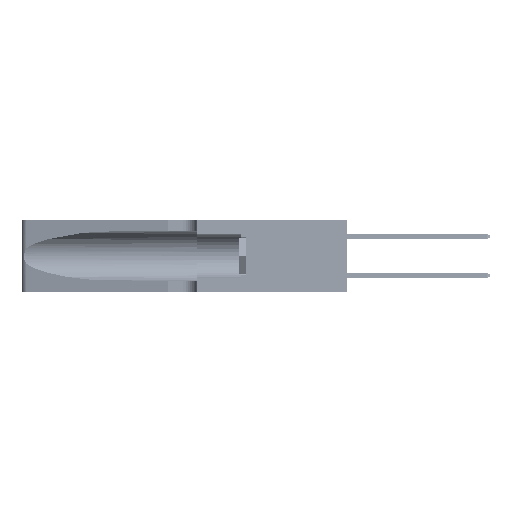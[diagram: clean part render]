
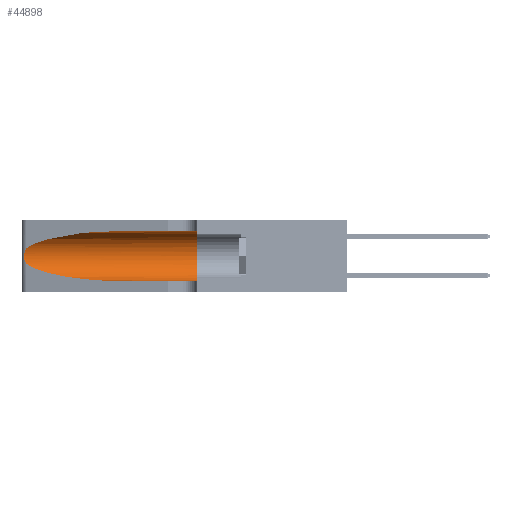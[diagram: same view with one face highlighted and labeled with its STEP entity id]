
A CAD part, left-side view. The second image highlights one B-rep face of the part: STEP entity #44898.
In plain terms, the highlighted cylindrical face has radius 3.308 mm (diameter 6.617 mm), a partial arc.
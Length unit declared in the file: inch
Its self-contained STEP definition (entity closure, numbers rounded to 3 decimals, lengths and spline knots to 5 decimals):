
#579 = CARTESIAN_POINT ( 'NONE',  ( 0.25487, 1.22718, 0.14631 ) ) ;
#1348 = CARTESIAN_POINT ( 'NONE',  ( 0.25487, 1.22718, 0.14631 ) ) ;
#1531 = CARTESIAN_POINT ( 'NONE',  ( 0.25639, 1.23184, 0.21858 ) ) ;
#1665 = EDGE_CURVE ( 'NONE', #18234, #7798, #29193, .T. ) ;
#2332 = ORIENTED_EDGE ( 'NONE', *, *, #12130, .F. ) ;
#2845 = CYLINDRICAL_SURFACE ( 'NONE', #19624, 0.13025 ) ;
#4830 = DIRECTION ( 'NONE',  ( 0., 1., 0. ) ) ;
#4990 = EDGE_CURVE ( 'NONE', #44279, #20820, #53232, .T. ) ;
#7434 = CARTESIAN_POINT ( 'NONE',  ( 0.1305, 1.61858, 0.185 ) ) ;
#7798 = VERTEX_POINT ( 'NONE', #15368 ) ;
#9820 = CARTESIAN_POINT ( 'NONE',  ( 0.26018, 1.23835, 0.19895 ) ) ;
#10367 = CARTESIAN_POINT ( 'NONE',  ( 0.1305, 0.35, 0.31525 ) ) ;
#10789 = CARTESIAN_POINT ( 'NONE',  ( 0.1305, 1.61858, 0.05475 ) ) ;
#12130 = EDGE_CURVE ( 'NONE', #43052, #50158, #14199, .T. ) ;
#13194 = CARTESIAN_POINT ( 'NONE',  ( 0.2373, 1.15595, 0.08982 ) ) ;
#13566 = CARTESIAN_POINT ( 'NONE',  ( 0.1305, 0.72297, 0.31525 ) ) ;
#13783 = CARTESIAN_POINT ( 'NONE',  ( 0.25487, 1.22718, 0.22369 ) ) ;
#14199 = CIRCLE ( 'NONE', #18807, 0.13025 ) ;
#14729 = CARTESIAN_POINT ( 'NONE',  ( 0.1305, 0.72297, 0.31525 ) ) ;
#15368 = CARTESIAN_POINT ( 'NONE',  ( 0.1305, 0.72297, 0.05475 ) ) ;
#15541 = DIRECTION ( 'NONE',  ( 0., -1., 0. ) ) ;
#16597 = CARTESIAN_POINT ( 'NONE',  ( 0.25487, 1.22718, 0.22369 ) ) ;
#17416 = DIRECTION ( 'NONE',  ( 0., 0., 1. ) ) ;
#17574 = CARTESIAN_POINT ( 'NONE',  ( 0.26075, 1.23896, 0.178 ) ) ;
#17722 = CARTESIAN_POINT ( 'NONE',  ( 0.25487, 1.22718, 0.22369 ) ) ;
#17748 = CARTESIAN_POINT ( 'NONE',  ( 0.25555, 1.22994, 0.2215 ) ) ;
#18069 = VECTOR ( 'NONE', #27787, 39.37008 ) ;
#18234 = VERTEX_POINT ( 'NONE', #23563 ) ;
#18807 = AXIS2_PLACEMENT_3D ( 'NONE', #29470, #4830, #17416 ) ;
#19624 = AXIS2_PLACEMENT_3D ( 'NONE', #7434, #15541, #19695 ) ;
#19695 = DIRECTION ( 'NONE',  ( 0., 0., -1. ) ) ;
#20820 = VERTEX_POINT ( 'NONE', #16597 ) ;
#21544 = CARTESIAN_POINT ( 'NONE',  ( 0.26017, 1.23833, 0.17102 ) ) ;
#21895 = CARTESIAN_POINT ( 'NONE',  ( 0.25787, 1.23484, 0.2124 ) ) ;
#21981 = B_SPLINE_CURVE_WITH_KNOTS ( 'NONE', 3,
 ( #13783, #17748, #1531, #21895, #30318, #9820, #42893, #17574, #21544, #26024, #38576, #46845, #25660, #1348 ),
 .UNSPECIFIED., .F., .F.,
 ( 4, 2, 2, 2, 2, 2, 4 ),
 ( 0., 0.00027, 0.00053, 0.00107, 0.0016, 0.00187, 0.00214 ),
 .UNSPECIFIED. ) ;
#23563 = CARTESIAN_POINT ( 'NONE',  ( 0.25487, 1.22718, 0.14631 ) ) ;
#23798 = ORIENTED_EDGE ( 'NONE', *, *, #26952, .T. ) ;
#24834 = EDGE_CURVE ( 'NONE', #7798, #50158, #39617, .T. ) ;
#25602 = CARTESIAN_POINT ( 'NONE',  ( 0.1305, 0.72297, 0.05475 ) ) ;
#25660 = CARTESIAN_POINT ( 'NONE',  ( 0.25555, 1.22993, 0.14849 ) ) ;
#26024 = CARTESIAN_POINT ( 'NONE',  ( 0.25856, 1.23593, 0.16098 ) ) ;
#26169 = CARTESIAN_POINT ( 'NONE',  ( 0.2373, 1.15595, 0.28018 ) ) ;
#26952 = EDGE_CURVE ( 'NONE', #20820, #18234, #21981, .T. ) ;
#27393 = CARTESIAN_POINT ( 'NONE',  ( 0.1305, 0.35, 0.05475 ) ) ;
#27787 = DIRECTION ( 'NONE',  ( 0., -1., 0. ) ) ;
#29193 =( BOUNDED_CURVE ( )  B_SPLINE_CURVE ( 3, ( #579, #13194, #37449, #25602 ),
 .UNSPECIFIED., .F., .F. ) 
 B_SPLINE_CURVE_WITH_KNOTS ( ( 4, 4 ),
 ( 3.44316, 4.71239 ),
 .UNSPECIFIED. ) 
 CURVE ( )  GEOMETRIC_REPRESENTATION_ITEM ( )  RATIONAL_B_SPLINE_CURVE ( ( 1., 0.87, 0.87, 1. ) ) 
 REPRESENTATION_ITEM ( '' )  );
#29470 = CARTESIAN_POINT ( 'NONE',  ( 0.1305, 0.35, 0.185 ) ) ;
#30010 = ORIENTED_EDGE ( 'NONE', *, *, #4990, .T. ) ;
#30318 = CARTESIAN_POINT ( 'NONE',  ( 0.25854, 1.2359, 0.20912 ) ) ;
#30445 = ORIENTED_EDGE ( 'NONE', *, *, #24834, .T. ) ;
#31321 = ORIENTED_EDGE ( 'NONE', *, *, #1665, .T. ) ;
#33232 = VECTOR ( 'NONE', #39541, 39.37008 ) ;
#34581 = EDGE_LOOP ( 'NONE', ( #30010, #23798, #31321, #30445, #2332, #50676 ) ) ;
#35658 = FACE_OUTER_BOUND ( 'NONE', #34581, .T. ) ;
#37449 = CARTESIAN_POINT ( 'NONE',  ( 0.18966, 0.96281, 0.05475 ) ) ;
#38192 = CARTESIAN_POINT ( 'NONE',  ( 0.18966, 0.96281, 0.31525 ) ) ;
#38576 = CARTESIAN_POINT ( 'NONE',  ( 0.25789, 1.23486, 0.15765 ) ) ;
#39541 = DIRECTION ( 'NONE',  ( 0., -1., 0. ) ) ;
#39617 = LINE ( 'NONE', #10789, #33232 ) ;
#42893 = CARTESIAN_POINT ( 'NONE',  ( 0.26075, 1.23896, 0.19203 ) ) ;
#43052 = VERTEX_POINT ( 'NONE', #10367 ) ;
#44279 = VERTEX_POINT ( 'NONE', #14729 ) ;
#44898 = ADVANCED_FACE ( 'NONE', ( #35658 ), #2845, .F. ) ;
#46845 = CARTESIAN_POINT ( 'NONE',  ( 0.25639, 1.23186, 0.15144 ) ) ;
#46978 = LINE ( 'NONE', #48251, #18069 ) ;
#48251 = CARTESIAN_POINT ( 'NONE',  ( 0.1305, 1.61858, 0.31525 ) ) ;
#49736 = EDGE_CURVE ( 'NONE', #44279, #43052, #46978, .T. ) ;
#50158 = VERTEX_POINT ( 'NONE', #27393 ) ;
#50676 = ORIENTED_EDGE ( 'NONE', *, *, #49736, .F. ) ;
#53232 =( BOUNDED_CURVE ( )  B_SPLINE_CURVE ( 3, ( #13566, #38192, #26169, #17722 ),
 .UNSPECIFIED., .F., .T. ) 
 B_SPLINE_CURVE_WITH_KNOTS ( ( 4, 4 ),
 ( 1.5708, 2.84003 ),
 .UNSPECIFIED. ) 
 CURVE ( )  GEOMETRIC_REPRESENTATION_ITEM ( )  RATIONAL_B_SPLINE_CURVE ( ( 1., 0.87, 0.87, 1. ) ) 
 REPRESENTATION_ITEM ( '' )  );
